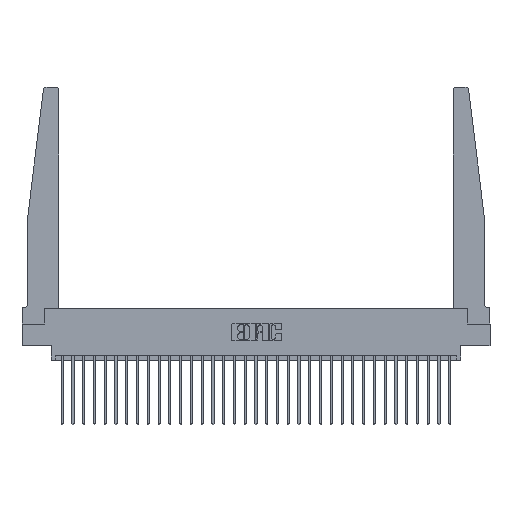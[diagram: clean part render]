
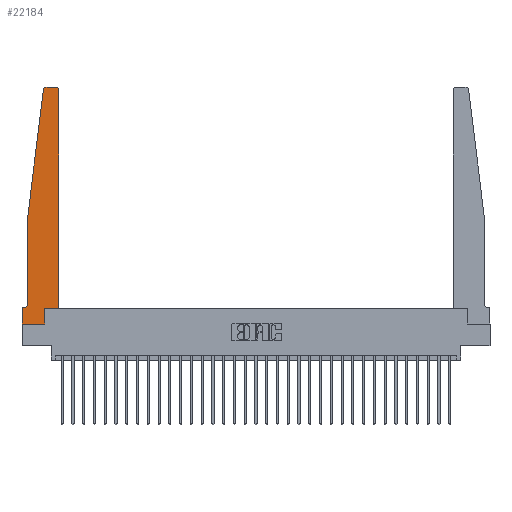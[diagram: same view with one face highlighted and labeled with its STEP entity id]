
A CAD part, top view. The second image highlights one B-rep face of the part: STEP entity #22184.
In plain terms, the highlighted planar face has unit normal (0, 0, 1).
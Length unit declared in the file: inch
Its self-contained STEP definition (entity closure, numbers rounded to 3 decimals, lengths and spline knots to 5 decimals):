
#129 = VERTEX_POINT ( 'NONE', #11720 ) ;
#187 = DIRECTION ( 'NONE',  ( 1., 0., 0. ) ) ;
#248 = LINE ( 'NONE', #18888, #4826 ) ;
#340 = LINE ( 'NONE', #20666, #20968 ) ;
#509 = ORIENTED_EDGE ( 'NONE', *, *, #24889, .T. ) ;
#690 = LINE ( 'NONE', #12011, #23877 ) ;
#901 = ORIENTED_EDGE ( 'NONE', *, *, #24053, .T. ) ;
#974 = EDGE_CURVE ( 'NONE', #129, #16430, #340, .T. ) ;
#1168 = ORIENTED_EDGE ( 'NONE', *, *, #23274, .T. ) ;
#1457 = CARTESIAN_POINT ( 'NONE',  ( 0.24675, 2.72367, 0.37 ) ) ;
#1496 = DIRECTION ( 'NONE',  ( 0., 1., 0. ) ) ;
#2014 = LINE ( 'NONE', #25099, #2452 ) ;
#2370 = EDGE_CURVE ( 'NONE', #20365, #20290, #27877, .T. ) ;
#2407 = VERTEX_POINT ( 'NONE', #28162 ) ;
#2452 = VECTOR ( 'NONE', #27237, 39.37008 ) ;
#2965 = DIRECTION ( 'NONE',  ( 1., 0., 0. ) ) ;
#3614 = DIRECTION ( 'NONE',  ( 0., 0., 1. ) ) ;
#3977 = EDGE_CURVE ( 'NONE', #2407, #22017, #28912, .T. ) ;
#4826 = VECTOR ( 'NONE', #23925, 39.37008 ) ;
#5009 = DIRECTION ( 'NONE',  ( -1., 0., 0. ) ) ;
#5503 = ORIENTED_EDGE ( 'NONE', *, *, #974, .T. ) ;
#5553 = CARTESIAN_POINT ( 'NONE',  ( 0.425, 0.18, 0.37 ) ) ;
#6940 = EDGE_CURVE ( 'NONE', #7363, #20895, #9375, .T. ) ;
#7183 = AXIS2_PLACEMENT_3D ( 'NONE', #24555, #3614, #26990 ) ;
#7363 = VERTEX_POINT ( 'NONE', #28004 ) ;
#7416 = CARTESIAN_POINT ( 'NONE',  ( 0.425, 2.72, 0.37 ) ) ;
#8581 = AXIS2_PLACEMENT_3D ( 'NONE', #21605, #16879, #2965 ) ;
#8726 = VECTOR ( 'NONE', #24263, 39.37008 ) ;
#9142 = LINE ( 'NONE', #25674, #27235 ) ;
#9375 = LINE ( 'NONE', #16106, #25397 ) ;
#9454 = EDGE_CURVE ( 'NONE', #16430, #24095, #17392, .T. ) ;
#9478 = LINE ( 'NONE', #11937, #8726 ) ;
#10381 = ORIENTED_EDGE ( 'NONE', *, *, #24067, .T. ) ;
#11501 = EDGE_LOOP ( 'NONE', ( #1168, #13281, #12660, #901, #17609, #509, #10381, #13125, #24909, #5503, #21167, #15936 ) ) ;
#11650 = CARTESIAN_POINT ( 'NONE',  ( 0.27653, 2.72, 0.37 ) ) ;
#11720 = CARTESIAN_POINT ( 'NONE',  ( 0.2605, 0.18, 0.37 ) ) ;
#11937 = CARTESIAN_POINT ( 'NONE',  ( 0.065, 0.1875, 0.37 ) ) ;
#12011 = CARTESIAN_POINT ( 'NONE',  ( 0.065, 1.25, 0.37 ) ) ;
#12156 = CARTESIAN_POINT ( 'NONE',  ( 0.2605, 0.18, 0.37 ) ) ;
#12177 = CARTESIAN_POINT ( 'NONE',  ( 0.015, 0.1875, 0.37 ) ) ;
#12660 = ORIENTED_EDGE ( 'NONE', *, *, #26052, .T. ) ;
#13125 = ORIENTED_EDGE ( 'NONE', *, *, #6940, .T. ) ;
#13281 = ORIENTED_EDGE ( 'NONE', *, *, #2370, .T. ) ;
#14285 = CARTESIAN_POINT ( 'NONE',  ( 0.065, 1.25, 0.37 ) ) ;
#15257 = CARTESIAN_POINT ( 'NONE',  ( 0.425, 0.18, 0.37 ) ) ;
#15361 = VERTEX_POINT ( 'NONE', #27383 ) ;
#15740 = AXIS2_PLACEMENT_3D ( 'NONE', #21429, #26033, #16251 ) ;
#15936 = ORIENTED_EDGE ( 'NONE', *, *, #20659, .T. ) ;
#16106 = CARTESIAN_POINT ( 'NONE',  ( 0., 0., 0.37 ) ) ;
#16150 = AXIS2_PLACEMENT_3D ( 'NONE', #11650, #23425, #20818 ) ;
#16245 = FACE_OUTER_BOUND ( 'NONE', #11501, .T. ) ;
#16251 = DIRECTION ( 'NONE',  ( -1., 0., 0. ) ) ;
#16430 = VERTEX_POINT ( 'NONE', #5553 ) ;
#16752 = VECTOR ( 'NONE', #1496, 39.37008 ) ;
#16879 = DIRECTION ( 'NONE',  ( 0., 0., 1. ) ) ;
#17318 = CARTESIAN_POINT ( 'NONE',  ( 0.2605, 0., 0.37 ) ) ;
#17392 = LINE ( 'NONE', #15257, #16752 ) ;
#17609 = ORIENTED_EDGE ( 'NONE', *, *, #3977, .T. ) ;
#17795 = EDGE_CURVE ( 'NONE', #20895, #129, #28664, .T. ) ;
#18857 = DIRECTION ( 'NONE',  ( 1., 0., 0. ) ) ;
#18888 = CARTESIAN_POINT ( 'NONE',  ( 0., 0., 0.37 ) ) ;
#19275 = VECTOR ( 'NONE', #21470, 39.37008 ) ;
#19388 = VERTEX_POINT ( 'NONE', #14285 ) ;
#19492 = CARTESIAN_POINT ( 'NONE',  ( 0.27653, 2.75, 0.37 ) ) ;
#20290 = VERTEX_POINT ( 'NONE', #1457 ) ;
#20365 = VERTEX_POINT ( 'NONE', #19492 ) ;
#20659 = EDGE_CURVE ( 'NONE', #24095, #15361, #21826, .T. ) ;
#20666 = CARTESIAN_POINT ( 'NONE',  ( 0.425, 0.18, 0.37 ) ) ;
#20818 = DIRECTION ( 'NONE',  ( 1., 0., 0. ) ) ;
#20895 = VERTEX_POINT ( 'NONE', #17318 ) ;
#20968 = VECTOR ( 'NONE', #187, 39.37008 ) ;
#21167 = ORIENTED_EDGE ( 'NONE', *, *, #9454, .T. ) ;
#21429 = CARTESIAN_POINT ( 'NONE',  ( 0.015, 0.2375, 0.37 ) ) ;
#21470 = DIRECTION ( 'NONE',  ( 0., 1., 0. ) ) ;
#21605 = CARTESIAN_POINT ( 'NONE',  ( 0.395, 2.72, 0.37 ) ) ;
#21826 = CIRCLE ( 'NONE', #8581, 0.03 ) ;
#22017 = VERTEX_POINT ( 'NONE', #12177 ) ;
#22184 = ADVANCED_FACE ( 'NONE', ( #16245 ), #29849, .T. ) ;
#22725 = CARTESIAN_POINT ( 'NONE',  ( 0., 0.1875, 0.37 ) ) ;
#23274 = EDGE_CURVE ( 'NONE', #15361, #20365, #9142, .T. ) ;
#23425 = DIRECTION ( 'NONE',  ( 0., 0., 1. ) ) ;
#23877 = VECTOR ( 'NONE', #28070, 39.37008 ) ;
#23925 = DIRECTION ( 'NONE',  ( 0., -1., 0. ) ) ;
#24053 = EDGE_CURVE ( 'NONE', #19388, #2407, #690, .T. ) ;
#24067 = EDGE_CURVE ( 'NONE', #25237, #7363, #248, .T. ) ;
#24095 = VERTEX_POINT ( 'NONE', #7416 ) ;
#24263 = DIRECTION ( 'NONE',  ( -1., 0., 0. ) ) ;
#24555 = CARTESIAN_POINT ( 'NONE',  ( 0., 0.1875, 0.37 ) ) ;
#24889 = EDGE_CURVE ( 'NONE', #22017, #25237, #9478, .T. ) ;
#24909 = ORIENTED_EDGE ( 'NONE', *, *, #17795, .T. ) ;
#25099 = CARTESIAN_POINT ( 'NONE',  ( 0.065, 1.25, 0.37 ) ) ;
#25237 = VERTEX_POINT ( 'NONE', #22725 ) ;
#25397 = VECTOR ( 'NONE', #18857, 39.37008 ) ;
#25674 = CARTESIAN_POINT ( 'NONE',  ( 0.25, 2.75, 0.37 ) ) ;
#26033 = DIRECTION ( 'NONE',  ( 0., 0., -1. ) ) ;
#26052 = EDGE_CURVE ( 'NONE', #20290, #19388, #2014, .T. ) ;
#26990 = DIRECTION ( 'NONE',  ( 1., 0., 0. ) ) ;
#27235 = VECTOR ( 'NONE', #5009, 39.37008 ) ;
#27237 = DIRECTION ( 'NONE',  ( -0.122, -0.992, 0. ) ) ;
#27383 = CARTESIAN_POINT ( 'NONE',  ( 0.395, 2.75, 0.37 ) ) ;
#27877 = CIRCLE ( 'NONE', #16150, 0.03 ) ;
#28004 = CARTESIAN_POINT ( 'NONE',  ( 0., 0., 0.37 ) ) ;
#28070 = DIRECTION ( 'NONE',  ( 0., -1., 0. ) ) ;
#28162 = CARTESIAN_POINT ( 'NONE',  ( 0.065, 0.2375, 0.37 ) ) ;
#28664 = LINE ( 'NONE', #12156, #19275 ) ;
#28912 = CIRCLE ( 'NONE', #15740, 0.05 ) ;
#29849 = PLANE ( 'NONE',  #7183 ) ;
